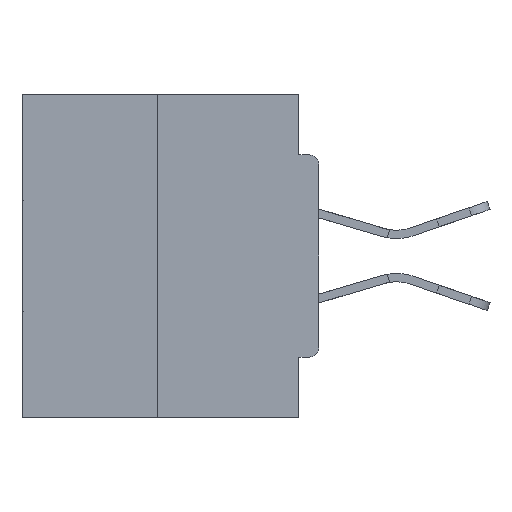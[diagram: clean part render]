
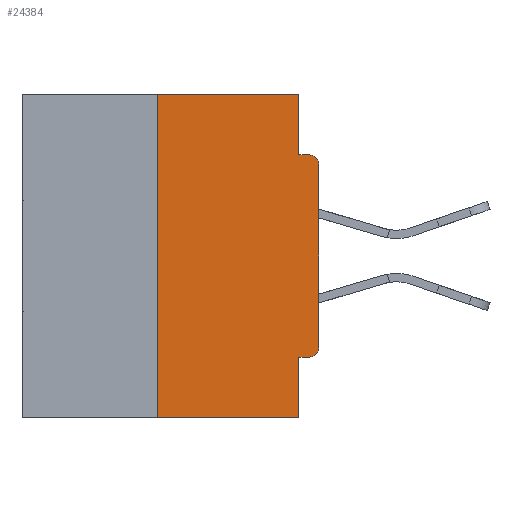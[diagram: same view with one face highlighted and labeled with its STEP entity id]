
A CAD part, left-side view. The second image highlights one B-rep face of the part: STEP entity #24384.
In plain terms, the highlighted planar face has unit normal (-1, 0, 0).
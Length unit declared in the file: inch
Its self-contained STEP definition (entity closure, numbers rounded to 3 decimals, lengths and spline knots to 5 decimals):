
#1012 = LINE ( 'NONE', #36335, #35160 ) ;
#1492 = ORIENTED_EDGE ( 'NONE', *, *, #25037, .F. ) ;
#1586 = DIRECTION ( 'NONE',  ( 0., 0., 1. ) ) ;
#1799 = DIRECTION ( 'NONE',  ( 0., -1., 0. ) ) ;
#2004 = ORIENTED_EDGE ( 'NONE', *, *, #38147, .F. ) ;
#3765 = CARTESIAN_POINT ( 'NONE',  ( 0., 0., -0.1085 ) ) ;
#5036 = VECTOR ( 'NONE', #17247, 39.37008 ) ;
#5611 = DIRECTION ( 'NONE',  ( 0., -1., 0. ) ) ;
#6442 = CARTESIAN_POINT ( 'NONE',  ( 0., 0., -0.4065 ) ) ;
#6667 = EDGE_CURVE ( 'NONE', #28587, #20072, #32333, .T. ) ;
#7096 = LINE ( 'NONE', #28915, #29394 ) ;
#7126 = VERTEX_POINT ( 'NONE', #32009 ) ;
#7679 = EDGE_CURVE ( 'NONE', #32886, #7126, #22649, .T. ) ;
#7680 = CARTESIAN_POINT ( 'NONE',  ( 0., 0., -0.0935 ) ) ;
#7903 = VECTOR ( 'NONE', #10711, 39.37008 ) ;
#7979 = CARTESIAN_POINT ( 'NONE',  ( 0., 0.031, -0.5 ) ) ;
#8326 = EDGE_CURVE ( 'NONE', #38616, #28587, #18835, .T. ) ;
#9128 = VERTEX_POINT ( 'NONE', #35057 ) ;
#9632 = DIRECTION ( 'NONE',  ( 0., 0., -1. ) ) ;
#9826 = VECTOR ( 'NONE', #1586, 39.37008 ) ;
#10711 = DIRECTION ( 'NONE',  ( 0., -1., 0. ) ) ;
#11360 = ORIENTED_EDGE ( 'NONE', *, *, #30324, .F. ) ;
#12192 = CARTESIAN_POINT ( 'NONE',  ( 0., 0.46, -0.5 ) ) ;
#12514 = DIRECTION ( 'NONE',  ( 0., 1., 0. ) ) ;
#12926 = ORIENTED_EDGE ( 'NONE', *, *, #15573, .F. ) ;
#13250 = CARTESIAN_POINT ( 'NONE',  ( 0., 0.015, -0.0935 ) ) ;
#13615 = ORIENTED_EDGE ( 'NONE', *, *, #6667, .T. ) ;
#14264 = CARTESIAN_POINT ( 'NONE',  ( 0., 0.031, -0.0935 ) ) ;
#14454 = CIRCLE ( 'NONE', #29400, 0.015 ) ;
#14687 = EDGE_CURVE ( 'NONE', #33714, #38616, #14454, .T. ) ;
#14990 = ORIENTED_EDGE ( 'NONE', *, *, #14687, .T. ) ;
#15396 = DIRECTION ( 'NONE',  ( 0., 0., -1. ) ) ;
#15440 = CARTESIAN_POINT ( 'NONE',  ( 0., 0.015, -0.4065 ) ) ;
#15573 = EDGE_CURVE ( 'NONE', #33714, #37412, #22445, .T. ) ;
#16853 = CARTESIAN_POINT ( 'NONE',  ( 0., 0., -0.3915 ) ) ;
#17247 = DIRECTION ( 'NONE',  ( 0., 0., -1. ) ) ;
#18511 = PLANE ( 'NONE',  #26578 ) ;
#18835 = LINE ( 'NONE', #28461, #9826 ) ;
#20072 = VERTEX_POINT ( 'NONE', #13250 ) ;
#21175 = VERTEX_POINT ( 'NONE', #25705 ) ;
#21690 = DIRECTION ( 'NONE',  ( -1., 0., 0. ) ) ;
#22151 = DIRECTION ( 'NONE',  ( 0., 0., 1. ) ) ;
#22445 = LINE ( 'NONE', #6442, #29356 ) ;
#22578 = LINE ( 'NONE', #7680, #7903 ) ;
#22635 = ORIENTED_EDGE ( 'NONE', *, *, #28431, .F. ) ;
#22649 = LINE ( 'NONE', #37404, #24559 ) ;
#24343 = VERTEX_POINT ( 'NONE', #14264 ) ;
#24384 = ADVANCED_FACE ( 'NONE', ( #36727 ), #18511, .F. ) ;
#24559 = VECTOR ( 'NONE', #22151, 39.37008 ) ;
#25037 = EDGE_CURVE ( 'NONE', #9128, #24343, #1012, .T. ) ;
#25705 = CARTESIAN_POINT ( 'NONE',  ( 0., 0.031, -0.5 ) ) ;
#26155 = EDGE_CURVE ( 'NONE', #32886, #21175, #26932, .T. ) ;
#26578 = AXIS2_PLACEMENT_3D ( 'NONE', #28066, #33568, #28462 ) ;
#26654 = DIRECTION ( 'NONE',  ( 0., 0., -1. ) ) ;
#26825 = CARTESIAN_POINT ( 'NONE',  ( 0., 0.25, -0.5 ) ) ;
#26932 = LINE ( 'NONE', #12192, #31732 ) ;
#28066 = CARTESIAN_POINT ( 'NONE',  ( 0., 0.46, 0. ) ) ;
#28431 = EDGE_CURVE ( 'NONE', #7126, #9128, #7096, .T. ) ;
#28461 = CARTESIAN_POINT ( 'NONE',  ( 0., 0., 0. ) ) ;
#28462 = DIRECTION ( 'NONE',  ( 0., 0., -1. ) ) ;
#28587 = VERTEX_POINT ( 'NONE', #3765 ) ;
#28915 = CARTESIAN_POINT ( 'NONE',  ( 0., 0.46, 0. ) ) ;
#29198 = ORIENTED_EDGE ( 'NONE', *, *, #8326, .T. ) ;
#29356 = VECTOR ( 'NONE', #12514, 39.37008 ) ;
#29394 = VECTOR ( 'NONE', #1799, 39.37008 ) ;
#29400 = AXIS2_PLACEMENT_3D ( 'NONE', #30760, #21690, #9632 ) ;
#30193 = LINE ( 'NONE', #7979, #5036 ) ;
#30324 = EDGE_CURVE ( 'NONE', #37412, #21175, #30193, .T. ) ;
#30760 = CARTESIAN_POINT ( 'NONE',  ( 0., 0.015, -0.3915 ) ) ;
#31732 = VECTOR ( 'NONE', #5611, 39.37008 ) ;
#32009 = CARTESIAN_POINT ( 'NONE',  ( 0., 0.25, 0. ) ) ;
#32071 = AXIS2_PLACEMENT_3D ( 'NONE', #39125, #33255, #26654 ) ;
#32333 = CIRCLE ( 'NONE', #32071, 0.015 ) ;
#32886 = VERTEX_POINT ( 'NONE', #26825 ) ;
#33255 = DIRECTION ( 'NONE',  ( -1., 0., 0. ) ) ;
#33568 = DIRECTION ( 'NONE',  ( 1., 0., 0. ) ) ;
#33714 = VERTEX_POINT ( 'NONE', #15440 ) ;
#34356 = EDGE_LOOP ( 'NONE', ( #22635, #34810, #36678, #11360, #12926, #14990, #29198, #13615, #2004, #1492 ) ) ;
#34810 = ORIENTED_EDGE ( 'NONE', *, *, #7679, .F. ) ;
#35057 = CARTESIAN_POINT ( 'NONE',  ( 0., 0.031, 0. ) ) ;
#35160 = VECTOR ( 'NONE', #15396, 39.37008 ) ;
#36335 = CARTESIAN_POINT ( 'NONE',  ( 0., 0.031, 0. ) ) ;
#36678 = ORIENTED_EDGE ( 'NONE', *, *, #26155, .T. ) ;
#36727 = FACE_OUTER_BOUND ( 'NONE', #34356, .T. ) ;
#37404 = CARTESIAN_POINT ( 'NONE',  ( 0., 0.25, 0. ) ) ;
#37412 = VERTEX_POINT ( 'NONE', #37622 ) ;
#37622 = CARTESIAN_POINT ( 'NONE',  ( 0., 0.031, -0.4065 ) ) ;
#38147 = EDGE_CURVE ( 'NONE', #24343, #20072, #22578, .T. ) ;
#38616 = VERTEX_POINT ( 'NONE', #16853 ) ;
#39125 = CARTESIAN_POINT ( 'NONE',  ( 0., 0.015, -0.1085 ) ) ;
